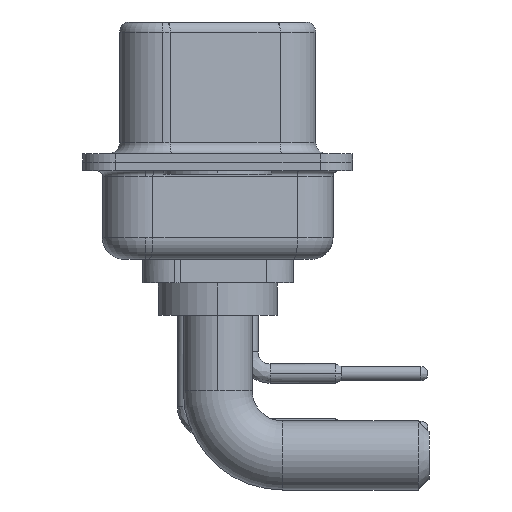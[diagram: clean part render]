
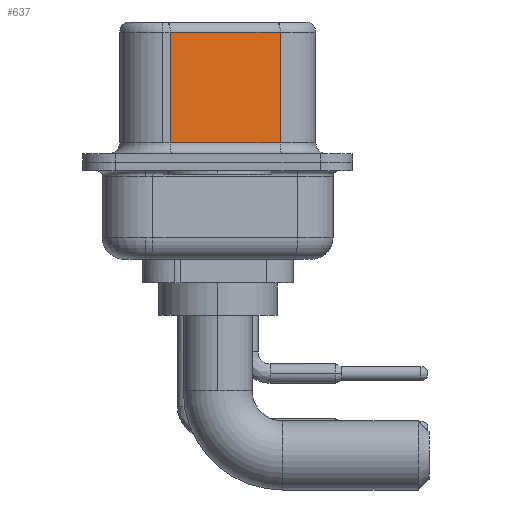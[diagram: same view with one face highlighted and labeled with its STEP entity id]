
A CAD part, left-side view. The second image highlights one B-rep face of the part: STEP entity #637.
In plain terms, the highlighted planar face has unit normal (-0.985, -0.174, 0).
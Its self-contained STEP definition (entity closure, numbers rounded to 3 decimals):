
#158 = LINE ( 'NONE', #3818, #14751 ) ;
#364 = DIRECTION ( 'NONE',  ( -0.174, 0.985, 0. ) ) ;
#637 = ADVANCED_FACE ( 'NONE', ( #11749 ), #17660, .F. ) ;
#639 = ORIENTED_EDGE ( 'NONE', *, *, #11542, .T. ) ;
#1069 = LINE ( 'NONE', #18385, #10049 ) ;
#2693 = ORIENTED_EDGE ( 'NONE', *, *, #22151, .F. ) ;
#3818 = CARTESIAN_POINT ( 'NONE',  ( 4.58, -2.897, 6.02 ) ) ;
#4168 = CARTESIAN_POINT ( 'NONE',  ( 4.58, -2.897, 6.52 ) ) ;
#4228 = EDGE_CURVE ( 'NONE', #12039, #13406, #18217, .T. ) ;
#5865 = AXIS2_PLACEMENT_3D ( 'NONE', #4168, #19564, #364 ) ;
#5914 = CARTESIAN_POINT ( 'NONE',  ( 4.58, -2.897, 0.9 ) ) ;
#6332 = CARTESIAN_POINT ( 'NONE',  ( 3.68, 2.203, 6.02 ) ) ;
#6775 = DIRECTION ( 'NONE',  ( 0., 0., -1. ) ) ;
#6793 = VECTOR ( 'NONE', #20800, 1000. ) ;
#7092 = DIRECTION ( 'NONE',  ( 0., 0., -1. ) ) ;
#7765 = VERTEX_POINT ( 'NONE', #7964 ) ;
#7964 = CARTESIAN_POINT ( 'NONE',  ( 4.58, -2.897, 6.02 ) ) ;
#9151 = ORIENTED_EDGE ( 'NONE', *, *, #9712, .T. ) ;
#9712 = EDGE_CURVE ( 'NONE', #7765, #12039, #158, .T. ) ;
#10049 = VECTOR ( 'NONE', #6775, 1000. ) ;
#11542 = EDGE_CURVE ( 'NONE', #13406, #19096, #14373, .T. ) ;
#11749 = FACE_OUTER_BOUND ( 'NONE', #21162, .T. ) ;
#12039 = VERTEX_POINT ( 'NONE', #6332 ) ;
#13406 = VERTEX_POINT ( 'NONE', #17389 ) ;
#14367 = ORIENTED_EDGE ( 'NONE', *, *, #4228, .T. ) ;
#14373 = LINE ( 'NONE', #19269, #6793 ) ;
#14751 = VECTOR ( 'NONE', #19231, 1000. ) ;
#17389 = CARTESIAN_POINT ( 'NONE',  ( 3.68, 2.203, 0.9 ) ) ;
#17660 = PLANE ( 'NONE',  #5865 ) ;
#18217 = LINE ( 'NONE', #24024, #22218 ) ;
#18385 = CARTESIAN_POINT ( 'NONE',  ( 4.58, -2.897, 6.52 ) ) ;
#19096 = VERTEX_POINT ( 'NONE', #5914 ) ;
#19231 = DIRECTION ( 'NONE',  ( -0.174, 0.985, 0. ) ) ;
#19269 = CARTESIAN_POINT ( 'NONE',  ( 4.58, -2.897, 0.9 ) ) ;
#19564 = DIRECTION ( 'NONE',  ( 0.985, 0.174, 0. ) ) ;
#20800 = DIRECTION ( 'NONE',  ( 0.174, -0.985, 0. ) ) ;
#21162 = EDGE_LOOP ( 'NONE', ( #2693, #9151, #14367, #639 ) ) ;
#22151 = EDGE_CURVE ( 'NONE', #7765, #19096, #1069, .T. ) ;
#22218 = VECTOR ( 'NONE', #7092, 1000. ) ;
#24024 = CARTESIAN_POINT ( 'NONE',  ( 3.68, 2.203, 6.52 ) ) ;
